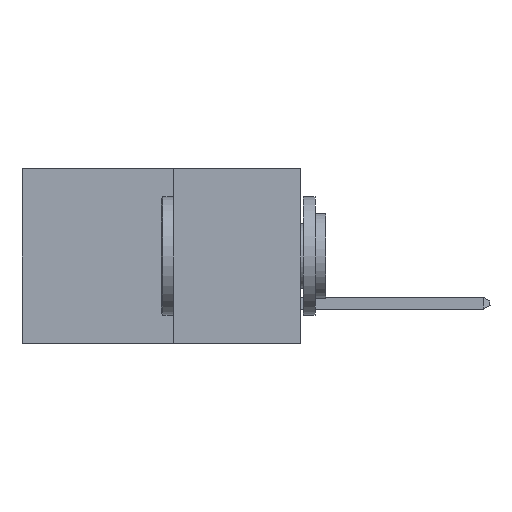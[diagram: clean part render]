
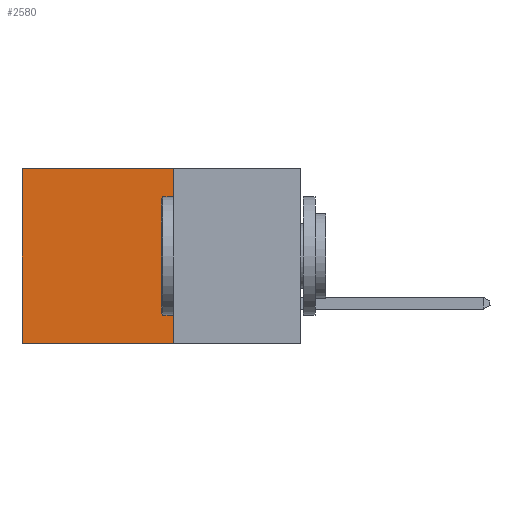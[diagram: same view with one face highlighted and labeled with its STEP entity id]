
A CAD part, left-side view. The second image highlights one B-rep face of the part: STEP entity #2580.
In plain terms, the highlighted planar face has unit normal (-1, 0, 0).
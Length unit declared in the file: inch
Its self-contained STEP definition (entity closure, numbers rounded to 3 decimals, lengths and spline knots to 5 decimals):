
#1025 = VERTEX_POINT ( 'NONE', #24254 ) ;
#1132 = VERTEX_POINT ( 'NONE', #13155 ) ;
#1607 = CARTESIAN_POINT ( 'NONE',  ( 0.277, 0.59, -0.37 ) ) ;
#2350 = CARTESIAN_POINT ( 'NONE',  ( 0.277, 0.27, -0.37 ) ) ;
#2580 = ADVANCED_FACE ( 'NONE', ( #7397 ), #5490, .F. ) ;
#3023 = CARTESIAN_POINT ( 'NONE',  ( 0.277, 0.27, -0.37 ) ) ;
#3044 = ORIENTED_EDGE ( 'NONE', *, *, #21800, .F. ) ;
#3369 = AXIS2_PLACEMENT_3D ( 'NONE', #5540, #5147, #5151 ) ;
#5147 = DIRECTION ( 'NONE',  ( 1., 0., 0. ) ) ;
#5151 = DIRECTION ( 'NONE',  ( 0., 0., -1. ) ) ;
#5490 = PLANE ( 'NONE',  #3369 ) ;
#5540 = CARTESIAN_POINT ( 'NONE',  ( 0.277, 0.27, -0.37 ) ) ;
#6559 = VECTOR ( 'NONE', #14931, 39.37008 ) ;
#7397 = FACE_OUTER_BOUND ( 'NONE', #11798, .T. ) ;
#9169 = VERTEX_POINT ( 'NONE', #27109 ) ;
#10837 = LINE ( 'NONE', #1607, #15768 ) ;
#11478 = LINE ( 'NONE', #2350, #15756 ) ;
#11798 = EDGE_LOOP ( 'NONE', ( #23343, #15293, #3044, #23755 ) ) ;
#13155 = CARTESIAN_POINT ( 'NONE',  ( 0.277, 0.27, -0.37 ) ) ;
#13905 = VERTEX_POINT ( 'NONE', #25491 ) ;
#14928 = VECTOR ( 'NONE', #22004, 39.37008 ) ;
#14931 = DIRECTION ( 'NONE',  ( 0., 1., 0. ) ) ;
#15070 = EDGE_CURVE ( 'NONE', #13905, #1025, #23348, .T. ) ;
#15293 = ORIENTED_EDGE ( 'NONE', *, *, #25102, .F. ) ;
#15570 = EDGE_CURVE ( 'NONE', #1025, #9169, #10837, .T. ) ;
#15596 = LINE ( 'NONE', #3023, #14928 ) ;
#15756 = VECTOR ( 'NONE', #25483, 39.37008 ) ;
#15768 = VECTOR ( 'NONE', #24600, 39.37008 ) ;
#19117 = CARTESIAN_POINT ( 'NONE',  ( 0.277, 0.27, 0. ) ) ;
#21800 = EDGE_CURVE ( 'NONE', #13905, #1132, #15596, .T. ) ;
#22004 = DIRECTION ( 'NONE',  ( 0., 0., -1. ) ) ;
#23343 = ORIENTED_EDGE ( 'NONE', *, *, #15570, .T. ) ;
#23348 = LINE ( 'NONE', #19117, #6559 ) ;
#23755 = ORIENTED_EDGE ( 'NONE', *, *, #15070, .T. ) ;
#24254 = CARTESIAN_POINT ( 'NONE',  ( 0.277, 0.59, 0. ) ) ;
#24600 = DIRECTION ( 'NONE',  ( 0., 0., -1. ) ) ;
#25102 = EDGE_CURVE ( 'NONE', #1132, #9169, #11478, .T. ) ;
#25483 = DIRECTION ( 'NONE',  ( 0., 1., 0. ) ) ;
#25491 = CARTESIAN_POINT ( 'NONE',  ( 0.277, 0.27, 0. ) ) ;
#27109 = CARTESIAN_POINT ( 'NONE',  ( 0.277, 0.59, -0.37 ) ) ;
